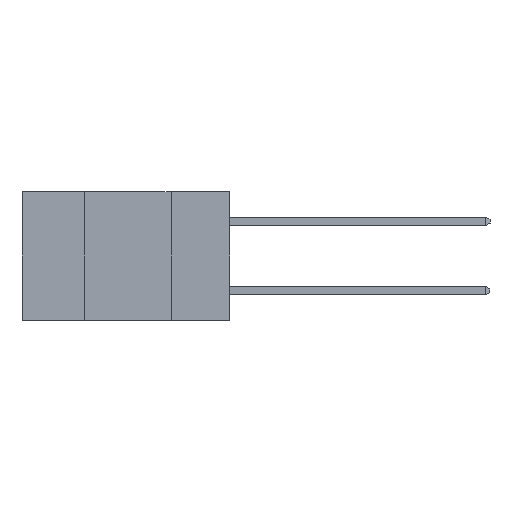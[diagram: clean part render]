
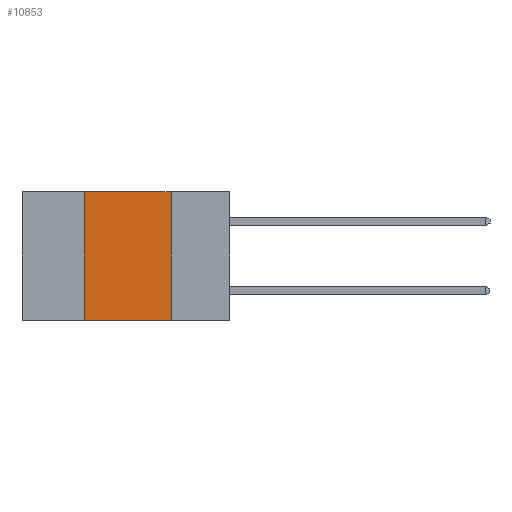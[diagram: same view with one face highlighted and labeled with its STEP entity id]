
A CAD part, left-side view. The second image highlights one B-rep face of the part: STEP entity #10853.
In plain terms, the highlighted planar face has unit normal (-1, 0, 0).
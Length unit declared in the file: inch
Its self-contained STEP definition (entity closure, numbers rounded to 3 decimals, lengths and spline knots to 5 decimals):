
#287 = VECTOR ( 'NONE', #982, 39.37008 ) ;
#355 = EDGE_CURVE ( 'NONE', #13273, #1229, #6650, .T. ) ;
#415 = EDGE_LOOP ( 'NONE', ( #3675, #7587, #3330, #10028 ) ) ;
#643 = DIRECTION ( 'NONE',  ( 1., 0., 0. ) ) ;
#910 = VECTOR ( 'NONE', #4662, 39.37008 ) ;
#982 = DIRECTION ( 'NONE',  ( 0., -1., 0. ) ) ;
#1229 = VERTEX_POINT ( 'NONE', #4520 ) ;
#1579 = CARTESIAN_POINT ( 'NONE',  ( 0., 0.17, 0. ) ) ;
#2024 = AXIS2_PLACEMENT_3D ( 'NONE', #12978, #643, #7914 ) ;
#2600 = EDGE_CURVE ( 'NONE', #4908, #13273, #4005, .T. ) ;
#3171 = EDGE_CURVE ( 'NONE', #4908, #4922, #5815, .T. ) ;
#3269 = DIRECTION ( 'NONE',  ( 0., -1., 0. ) ) ;
#3330 = ORIENTED_EDGE ( 'NONE', *, *, #2600, .F. ) ;
#3675 = ORIENTED_EDGE ( 'NONE', *, *, #9603, .F. ) ;
#4005 = LINE ( 'NONE', #5000, #910 ) ;
#4520 = CARTESIAN_POINT ( 'NONE',  ( 0., 0.17, 0. ) ) ;
#4662 = DIRECTION ( 'NONE',  ( 0., 0., 1. ) ) ;
#4908 = VERTEX_POINT ( 'NONE', #11435 ) ;
#4922 = VERTEX_POINT ( 'NONE', #6546 ) ;
#5000 = CARTESIAN_POINT ( 'NONE',  ( 0., 0.42, 0. ) ) ;
#5517 = CARTESIAN_POINT ( 'NONE',  ( 0., 0.42, 0. ) ) ;
#5605 = LINE ( 'NONE', #1579, #8050 ) ;
#5815 = LINE ( 'NONE', #7949, #287 ) ;
#5819 = PLANE ( 'NONE',  #2024 ) ;
#6057 = FACE_OUTER_BOUND ( 'NONE', #415, .T. ) ;
#6546 = CARTESIAN_POINT ( 'NONE',  ( 0., 0.17, -0.37 ) ) ;
#6650 = LINE ( 'NONE', #7769, #11758 ) ;
#7587 = ORIENTED_EDGE ( 'NONE', *, *, #355, .F. ) ;
#7769 = CARTESIAN_POINT ( 'NONE',  ( 0., 0.6, 0. ) ) ;
#7914 = DIRECTION ( 'NONE',  ( 0., 0., -1. ) ) ;
#7949 = CARTESIAN_POINT ( 'NONE',  ( 0., 0.6, -0.37 ) ) ;
#8050 = VECTOR ( 'NONE', #10874, 39.37008 ) ;
#9603 = EDGE_CURVE ( 'NONE', #1229, #4922, #5605, .T. ) ;
#10028 = ORIENTED_EDGE ( 'NONE', *, *, #3171, .T. ) ;
#10853 = ADVANCED_FACE ( 'NONE', ( #6057 ), #5819, .F. ) ;
#10874 = DIRECTION ( 'NONE',  ( 0., 0., -1. ) ) ;
#11435 = CARTESIAN_POINT ( 'NONE',  ( 0., 0.42, -0.37 ) ) ;
#11758 = VECTOR ( 'NONE', #3269, 39.37008 ) ;
#12978 = CARTESIAN_POINT ( 'NONE',  ( 0., 0.6, 0. ) ) ;
#13273 = VERTEX_POINT ( 'NONE', #5517 ) ;
